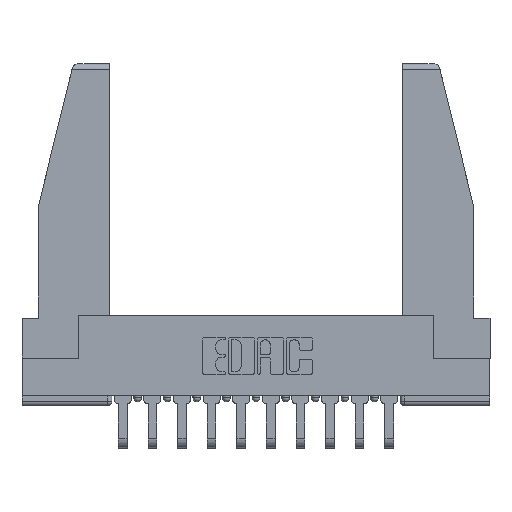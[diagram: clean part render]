
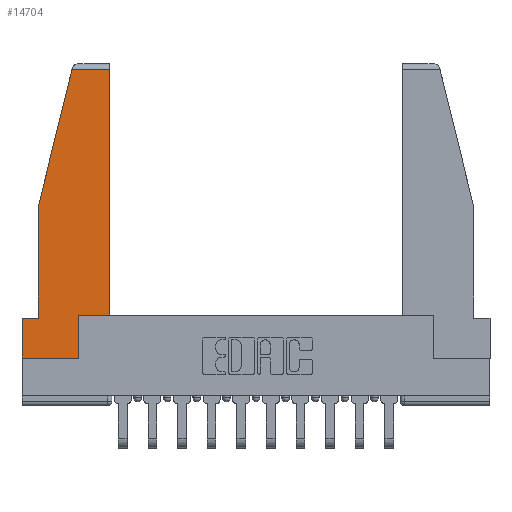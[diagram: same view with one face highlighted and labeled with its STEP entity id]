
A CAD part, top view. The second image highlights one B-rep face of the part: STEP entity #14704.
In plain terms, the highlighted planar face has unit normal (0, 0, 1).
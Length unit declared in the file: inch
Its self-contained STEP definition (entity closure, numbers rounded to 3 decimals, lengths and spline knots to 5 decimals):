
#81 = VECTOR ( 'NONE', #10667, 39.37008 ) ;
#253 = LINE ( 'NONE', #15590, #81 ) ;
#315 = CARTESIAN_POINT ( 'NONE',  ( 0.086, 0.8, 0. ) ) ;
#467 = VERTEX_POINT ( 'NONE', #13521 ) ;
#631 = DIRECTION ( 'NONE',  ( -0.239, -0.971, 0. ) ) ;
#713 = CARTESIAN_POINT ( 'NONE',  ( 0.297, 0., 0. ) ) ;
#718 = VERTEX_POINT ( 'NONE', #2054 ) ;
#1585 = ORIENTED_EDGE ( 'NONE', *, *, #4772, .T. ) ;
#1645 = CARTESIAN_POINT ( 'NONE',  ( 0., 1.52, 0. ) ) ;
#1879 = LINE ( 'NONE', #12544, #9989 ) ;
#2015 = ORIENTED_EDGE ( 'NONE', *, *, #3513, .T. ) ;
#2054 = CARTESIAN_POINT ( 'NONE',  ( 0., 0.21, 0. ) ) ;
#2139 = DIRECTION ( 'NONE',  ( 0., -1., 0. ) ) ;
#2585 = ORIENTED_EDGE ( 'NONE', *, *, #5537, .T. ) ;
#3090 = DIRECTION ( 'NONE',  ( -1., 0., 0. ) ) ;
#3513 = EDGE_CURVE ( 'NONE', #10751, #13618, #5805, .T. ) ;
#3799 = LINE ( 'NONE', #16661, #15408 ) ;
#4348 = LINE ( 'NONE', #13315, #11519 ) ;
#4560 = PLANE ( 'NONE',  #9265 ) ;
#4693 = VECTOR ( 'NONE', #631, 39.37008 ) ;
#4744 = VECTOR ( 'NONE', #6143, 39.37008 ) ;
#4768 = ORIENTED_EDGE ( 'NONE', *, *, #10416, .T. ) ;
#4772 = EDGE_CURVE ( 'NONE', #14528, #467, #3799, .T. ) ;
#4785 = LINE ( 'NONE', #13509, #4693 ) ;
#5211 = EDGE_CURVE ( 'NONE', #11604, #10751, #10030, .T. ) ;
#5537 = EDGE_CURVE ( 'NONE', #467, #718, #13398, .T. ) ;
#5805 = LINE ( 'NONE', #9786, #13733 ) ;
#5993 = DIRECTION ( 'NONE',  ( 0., 0., 1. ) ) ;
#6143 = DIRECTION ( 'NONE',  ( 1., 0., 0. ) ) ;
#6169 = CARTESIAN_POINT ( 'NONE',  ( 0., 0., 0. ) ) ;
#6661 = EDGE_LOOP ( 'NONE', ( #2015, #4768, #16697, #1585, #2585, #8476, #15356, #7980, #12624 ) ) ;
#6775 = EDGE_CURVE ( 'NONE', #11360, #11604, #4348, .T. ) ;
#6796 = VERTEX_POINT ( 'NONE', #10438 ) ;
#7759 = CARTESIAN_POINT ( 'NONE',  ( 0.2636, 1.52, 0. ) ) ;
#7980 = ORIENTED_EDGE ( 'NONE', *, *, #6775, .T. ) ;
#8476 = ORIENTED_EDGE ( 'NONE', *, *, #11043, .T. ) ;
#8541 = VERTEX_POINT ( 'NONE', #7759 ) ;
#8622 = VECTOR ( 'NONE', #3090, 39.37008 ) ;
#9265 = AXIS2_PLACEMENT_3D ( 'NONE', #6169, #5993, #12516 ) ;
#9353 = CARTESIAN_POINT ( 'NONE',  ( 0.461, 1.52, 0. ) ) ;
#9671 = CARTESIAN_POINT ( 'NONE',  ( 0., 0.21, 0. ) ) ;
#9786 = CARTESIAN_POINT ( 'NONE',  ( 0.461, 0.223, 0. ) ) ;
#9989 = VECTOR ( 'NONE', #2139, 39.37008 ) ;
#10030 = LINE ( 'NONE', #13993, #4744 ) ;
#10416 = EDGE_CURVE ( 'NONE', #13618, #8541, #13234, .T. ) ;
#10438 = CARTESIAN_POINT ( 'NONE',  ( 0., 0., 0. ) ) ;
#10667 = DIRECTION ( 'NONE',  ( 1., 0., 0. ) ) ;
#10751 = VERTEX_POINT ( 'NONE', #14216 ) ;
#10977 = FACE_OUTER_BOUND ( 'NONE', #6661, .T. ) ;
#11043 = EDGE_CURVE ( 'NONE', #718, #6796, #1879, .T. ) ;
#11229 = VECTOR ( 'NONE', #13564, 39.37008 ) ;
#11360 = VERTEX_POINT ( 'NONE', #713 ) ;
#11519 = VECTOR ( 'NONE', #12971, 39.37008 ) ;
#11604 = VERTEX_POINT ( 'NONE', #14491 ) ;
#11644 = DIRECTION ( 'NONE',  ( 0., -1., 0. ) ) ;
#12516 = DIRECTION ( 'NONE',  ( 1., 0., 0. ) ) ;
#12544 = CARTESIAN_POINT ( 'NONE',  ( 0., 0.21, 0. ) ) ;
#12624 = ORIENTED_EDGE ( 'NONE', *, *, #5211, .T. ) ;
#12971 = DIRECTION ( 'NONE',  ( 0., 1., 0. ) ) ;
#13234 = LINE ( 'NONE', #1645, #8622 ) ;
#13315 = CARTESIAN_POINT ( 'NONE',  ( 0.297, 0., 0. ) ) ;
#13398 = LINE ( 'NONE', #9671, #11229 ) ;
#13509 = CARTESIAN_POINT ( 'NONE',  ( 0.271, 1.55, 0. ) ) ;
#13521 = CARTESIAN_POINT ( 'NONE',  ( 0.086, 0.21, 0. ) ) ;
#13564 = DIRECTION ( 'NONE',  ( -1., 0., 0. ) ) ;
#13618 = VERTEX_POINT ( 'NONE', #9353 ) ;
#13733 = VECTOR ( 'NONE', #14946, 39.37008 ) ;
#13993 = CARTESIAN_POINT ( 'NONE',  ( 0.297, 0.223, 0. ) ) ;
#14216 = CARTESIAN_POINT ( 'NONE',  ( 0.461, 0.223, 0. ) ) ;
#14491 = CARTESIAN_POINT ( 'NONE',  ( 0.297, 0.223, 0. ) ) ;
#14528 = VERTEX_POINT ( 'NONE', #315 ) ;
#14704 = ADVANCED_FACE ( 'NONE', ( #10977 ), #4560, .T. ) ;
#14946 = DIRECTION ( 'NONE',  ( 0., 1., 0. ) ) ;
#15108 = EDGE_CURVE ( 'NONE', #8541, #14528, #4785, .T. ) ;
#15356 = ORIENTED_EDGE ( 'NONE', *, *, #15682, .T. ) ;
#15408 = VECTOR ( 'NONE', #11644, 39.37008 ) ;
#15590 = CARTESIAN_POINT ( 'NONE',  ( 0., 0., 0. ) ) ;
#15682 = EDGE_CURVE ( 'NONE', #6796, #11360, #253, .T. ) ;
#16661 = CARTESIAN_POINT ( 'NONE',  ( 0.086, 0.8, 0. ) ) ;
#16697 = ORIENTED_EDGE ( 'NONE', *, *, #15108, .T. ) ;
